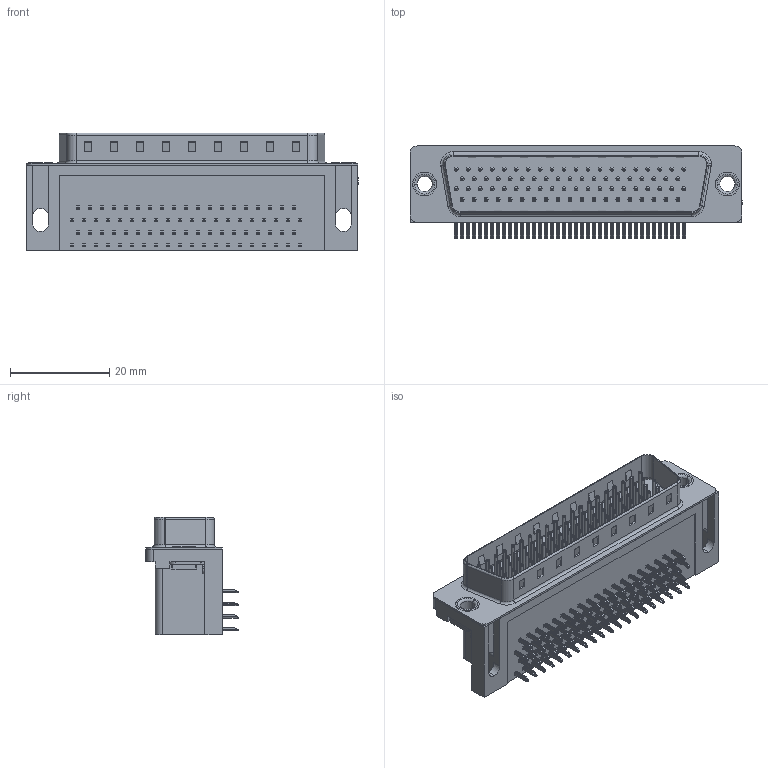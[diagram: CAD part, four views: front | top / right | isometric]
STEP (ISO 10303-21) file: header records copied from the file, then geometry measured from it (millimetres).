
FILE_DESCRIPTION (( 'STEP AP203' ), '1' );
FILE_NAME ('633-078-363-501.STEP', '2018-09-08T15:12:54', ( '' ), ( '' ), 'SwSTEP 2.0', 'SolidWorks 2016', '' );
FILE_SCHEMA (( 'CONFIG_CONTROL_DESIGN' ));
Length unit declared in the file: millimetre
Products named in the file (9): 633 Contact Bottom_78 Contact; 633 Contact Middle_78 Contact; 633 Contact Top_78 Contact; 633 Contact Top 78; 633 Non Board Mount_78 Contact; 633 Thru Hole Rivet; 633-078-363-501; 633 Housing_78 Contact; 633 Shell_78 Contact
Assembly tree (84 placements, depth 2):
  633-078-363-501
    633 Housing_78 Contact
    633 Shell_78 Contact
    633 Contact Bottom_78 Contact  x19
    633 Contact Middle_78 Contact  x20
    633 Contact Top_78 Contact  x19
    633 Contact Top 78  x20
    633 Non Board Mount_78 Contact  x2
    633 Thru Hole Rivet  x2
Bounding box: 67 x 18.58 x 23.8 mm (x, y, z)
Volume: 14553.5 mm3; surface area: 16105.6 mm2
Topology: 84 solids, 84 shells, 6230 faces, 15284 edges, 9385 vertices
Faces by surface type: plane 3979, cylinder 1756, torus 495
Entity records: 38933 total; most frequent: DIRECTION 6322, CARTESIAN_POINT 6229, ORIENTED_EDGE 5914, EDGE_CURVE 2957, VECTOR 2182, LINE 2182, AXIS2_PLACEMENT_3D 2070, VERTEX_POINT 1909
